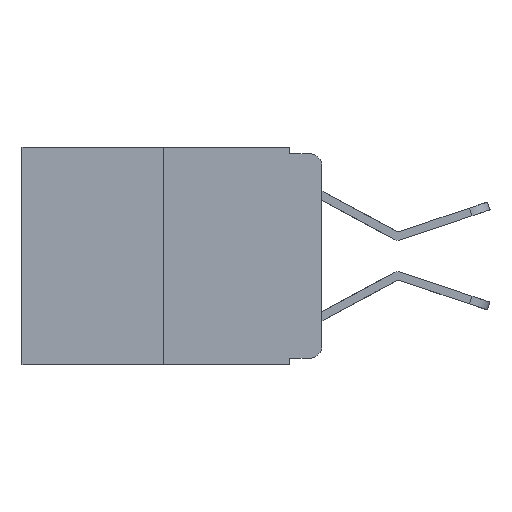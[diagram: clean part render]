
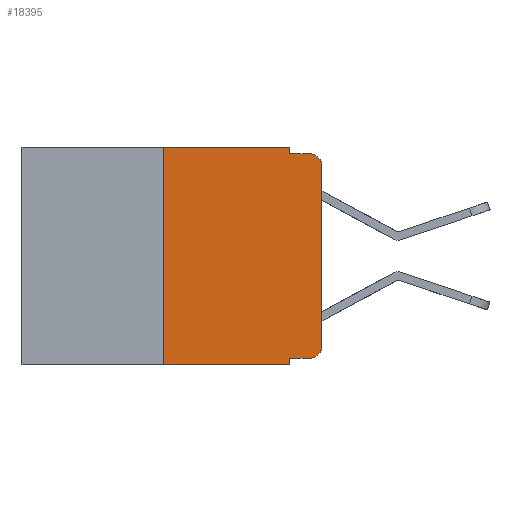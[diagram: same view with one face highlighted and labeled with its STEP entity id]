
A CAD part, left-side view. The second image highlights one B-rep face of the part: STEP entity #18395.
In plain terms, the highlighted planar face has unit normal (-1, 0, 0).
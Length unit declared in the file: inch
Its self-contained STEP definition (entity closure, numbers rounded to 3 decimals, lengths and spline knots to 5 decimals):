
#528 = LINE ( 'NONE', #4921, #18360 ) ;
#543 = EDGE_CURVE ( 'NONE', #4700, #10853, #2762, .T. ) ;
#885 = VERTEX_POINT ( 'NONE', #13411 ) ;
#1111 = EDGE_CURVE ( 'NONE', #10853, #8019, #528, .T. ) ;
#1512 = DIRECTION ( 'NONE',  ( 0., 0., -1. ) ) ;
#1697 = VECTOR ( 'NONE', #12709, 39.37008 ) ;
#1986 = VERTEX_POINT ( 'NONE', #19433 ) ;
#2224 = CARTESIAN_POINT ( 'NONE',  ( 0., 0.473, 0. ) ) ;
#2654 = LINE ( 'NONE', #12456, #20337 ) ;
#2762 = CIRCLE ( 'NONE', #11133, 0.02 ) ;
#3189 = ORIENTED_EDGE ( 'NONE', *, *, #3771, .F. ) ;
#3230 = CARTESIAN_POINT ( 'NONE',  ( 0., 0.25, 0. ) ) ;
#3317 = VECTOR ( 'NONE', #4025, 39.37008 ) ;
#3391 = VECTOR ( 'NONE', #8913, 39.37008 ) ;
#3742 = ORIENTED_EDGE ( 'NONE', *, *, #6078, .F. ) ;
#3771 = EDGE_CURVE ( 'NONE', #18805, #20941, #2654, .T. ) ;
#3832 = VERTEX_POINT ( 'NONE', #14674 ) ;
#4025 = DIRECTION ( 'NONE',  ( 0., 0., -1. ) ) ;
#4700 = VERTEX_POINT ( 'NONE', #20883 ) ;
#4921 = CARTESIAN_POINT ( 'NONE',  ( 0., 0., 0. ) ) ;
#5686 = DIRECTION ( 'NONE',  ( 0., -1., 0. ) ) ;
#5954 = VECTOR ( 'NONE', #5686, 39.37008 ) ;
#6078 = EDGE_CURVE ( 'NONE', #1986, #3832, #9299, .T. ) ;
#6142 = ORIENTED_EDGE ( 'NONE', *, *, #8840, .F. ) ;
#6527 = CARTESIAN_POINT ( 'NONE',  ( 0., 0.473, 0. ) ) ;
#7227 = CARTESIAN_POINT ( 'NONE',  ( 0., 0., -0.03 ) ) ;
#7309 = AXIS2_PLACEMENT_3D ( 'NONE', #6527, #18558, #8283 ) ;
#7598 = CARTESIAN_POINT ( 'NONE',  ( 0., 0.02, -0.01 ) ) ;
#7979 = EDGE_CURVE ( 'NONE', #885, #4700, #17272, .T. ) ;
#8019 = VERTEX_POINT ( 'NONE', #7227 ) ;
#8283 = DIRECTION ( 'NONE',  ( 0., 0., -1. ) ) ;
#8420 = VERTEX_POINT ( 'NONE', #19192 ) ;
#8525 = ORIENTED_EDGE ( 'NONE', *, *, #543, .T. ) ;
#8840 = EDGE_CURVE ( 'NONE', #20941, #19943, #10554, .T. ) ;
#8913 = DIRECTION ( 'NONE',  ( 0., -1., 0. ) ) ;
#9062 = ORIENTED_EDGE ( 'NONE', *, *, #18466, .T. ) ;
#9299 = LINE ( 'NONE', #3230, #1697 ) ;
#9562 = DIRECTION ( 'NONE',  ( 0., 0., 1. ) ) ;
#9648 = AXIS2_PLACEMENT_3D ( 'NONE', #21979, #11872, #1512 ) ;
#9848 = ORIENTED_EDGE ( 'NONE', *, *, #10211, .T. ) ;
#10211 = EDGE_CURVE ( 'NONE', #1986, #8420, #12567, .T. ) ;
#10554 = LINE ( 'NONE', #18036, #5954 ) ;
#10853 = VERTEX_POINT ( 'NONE', #13973 ) ;
#10900 = CARTESIAN_POINT ( 'NONE',  ( 0., 0.051, 0. ) ) ;
#11133 = AXIS2_PLACEMENT_3D ( 'NONE', #16114, #16122, #16160 ) ;
#11872 = DIRECTION ( 'NONE',  ( -1., 0., 0. ) ) ;
#12071 = CARTESIAN_POINT ( 'NONE',  ( 0., 0.051, -0.01 ) ) ;
#12456 = CARTESIAN_POINT ( 'NONE',  ( 0., 0.051, 0. ) ) ;
#12567 = LINE ( 'NONE', #20824, #3391 ) ;
#12616 = CARTESIAN_POINT ( 'NONE',  ( 0., 0.051, 0. ) ) ;
#12709 = DIRECTION ( 'NONE',  ( 0., 0., 1. ) ) ;
#13411 = CARTESIAN_POINT ( 'NONE',  ( 0., 0.051, -0.333 ) ) ;
#13973 = CARTESIAN_POINT ( 'NONE',  ( 0., 0., -0.313 ) ) ;
#14674 = CARTESIAN_POINT ( 'NONE',  ( 0., 0.25, 0. ) ) ;
#16076 = VECTOR ( 'NONE', #21077, 39.37008 ) ;
#16114 = CARTESIAN_POINT ( 'NONE',  ( 0., 0.02, -0.313 ) ) ;
#16122 = DIRECTION ( 'NONE',  ( -1., 0., 0. ) ) ;
#16160 = DIRECTION ( 'NONE',  ( 0., 0., -1. ) ) ;
#16823 = PLANE ( 'NONE',  #7309 ) ;
#16895 = DIRECTION ( 'NONE',  ( 0., 0., -1. ) ) ;
#17015 = ORIENTED_EDGE ( 'NONE', *, *, #20488, .F. ) ;
#17067 = ORIENTED_EDGE ( 'NONE', *, *, #7979, .T. ) ;
#17272 = LINE ( 'NONE', #22058, #22166 ) ;
#17565 = CIRCLE ( 'NONE', #9648, 0.02 ) ;
#17614 = EDGE_CURVE ( 'NONE', #885, #8420, #21980, .T. ) ;
#18036 = CARTESIAN_POINT ( 'NONE',  ( 0., 0.051, -0.01 ) ) ;
#18360 = VECTOR ( 'NONE', #9562, 39.37008 ) ;
#18395 = ADVANCED_FACE ( 'NONE', ( #19155 ), #16823, .F. ) ;
#18466 = EDGE_CURVE ( 'NONE', #8019, #19943, #17565, .T. ) ;
#18558 = DIRECTION ( 'NONE',  ( 1., 0., 0. ) ) ;
#18673 = ORIENTED_EDGE ( 'NONE', *, *, #17614, .F. ) ;
#18696 = EDGE_LOOP ( 'NONE', ( #21848, #9062, #6142, #3189, #17015, #3742, #9848, #18673, #17067, #8525 ) ) ;
#18791 = DIRECTION ( 'NONE',  ( 0., -1., 0. ) ) ;
#18805 = VERTEX_POINT ( 'NONE', #12616 ) ;
#19155 = FACE_OUTER_BOUND ( 'NONE', #18696, .T. ) ;
#19192 = CARTESIAN_POINT ( 'NONE',  ( 0., 0.051, -0.343 ) ) ;
#19433 = CARTESIAN_POINT ( 'NONE',  ( 0., 0.25, -0.343 ) ) ;
#19943 = VERTEX_POINT ( 'NONE', #7598 ) ;
#20337 = VECTOR ( 'NONE', #16895, 39.37008 ) ;
#20488 = EDGE_CURVE ( 'NONE', #3832, #18805, #20598, .T. ) ;
#20598 = LINE ( 'NONE', #2224, #16076 ) ;
#20824 = CARTESIAN_POINT ( 'NONE',  ( 0., 0.473, -0.343 ) ) ;
#20883 = CARTESIAN_POINT ( 'NONE',  ( 0., 0.02, -0.333 ) ) ;
#20941 = VERTEX_POINT ( 'NONE', #12071 ) ;
#21077 = DIRECTION ( 'NONE',  ( 0., -1., 0. ) ) ;
#21848 = ORIENTED_EDGE ( 'NONE', *, *, #1111, .T. ) ;
#21979 = CARTESIAN_POINT ( 'NONE',  ( 0., 0.02, -0.03 ) ) ;
#21980 = LINE ( 'NONE', #10900, #3317 ) ;
#22058 = CARTESIAN_POINT ( 'NONE',  ( 0., 0.051, -0.333 ) ) ;
#22166 = VECTOR ( 'NONE', #18791, 39.37008 ) ;
